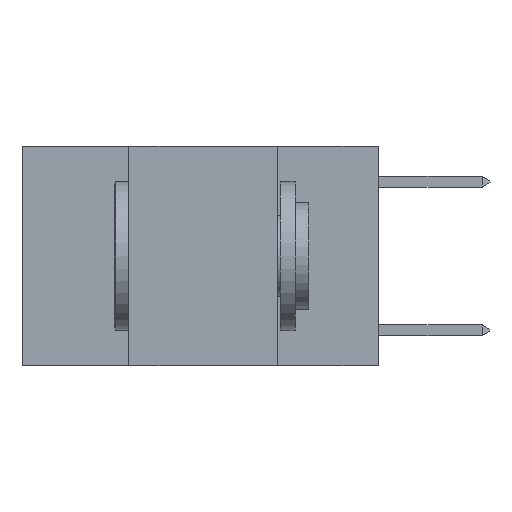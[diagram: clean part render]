
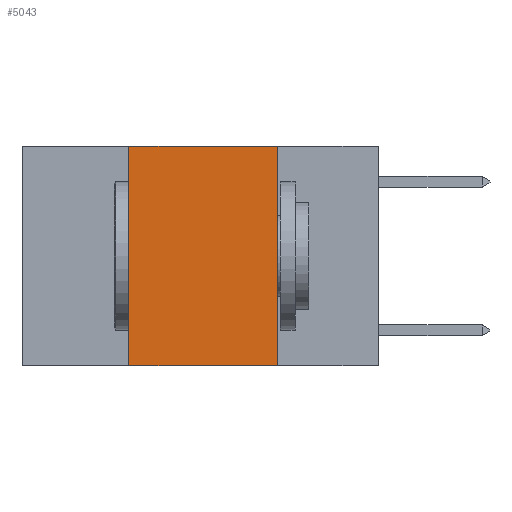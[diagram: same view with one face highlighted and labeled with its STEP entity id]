
A CAD part, left-side view. The second image highlights one B-rep face of the part: STEP entity #5043.
In plain terms, the highlighted planar face has unit normal (-1, 0, 0).
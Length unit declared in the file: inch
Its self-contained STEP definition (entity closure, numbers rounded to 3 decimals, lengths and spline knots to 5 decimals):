
#32 = VECTOR ( 'NONE', #8214, 39.37008 ) ;
#274 = CARTESIAN_POINT ( 'NONE',  ( 0., 0.6, 0. ) ) ;
#342 = VECTOR ( 'NONE', #1905, 39.37008 ) ;
#621 = EDGE_CURVE ( 'NONE', #5665, #5463, #1216, .T. ) ;
#1065 = CARTESIAN_POINT ( 'NONE',  ( 0., 0.42, -0.37 ) ) ;
#1211 = LINE ( 'NONE', #9480, #8311 ) ;
#1216 = LINE ( 'NONE', #7091, #3207 ) ;
#1454 = CARTESIAN_POINT ( 'NONE',  ( 0., 0.17, -0.37 ) ) ;
#1811 = DIRECTION ( 'NONE',  ( 1., 0., 0. ) ) ;
#1905 = DIRECTION ( 'NONE',  ( 0., -1., 0. ) ) ;
#2370 = ORIENTED_EDGE ( 'NONE', *, *, #3875, .F. ) ;
#3207 = VECTOR ( 'NONE', #4194, 39.37008 ) ;
#3368 = CARTESIAN_POINT ( 'NONE',  ( 0., 0.42, 0. ) ) ;
#3630 = ORIENTED_EDGE ( 'NONE', *, *, #9413, .T. ) ;
#3875 = EDGE_CURVE ( 'NONE', #6298, #5665, #1211, .T. ) ;
#4194 = DIRECTION ( 'NONE',  ( 0., -1., 0. ) ) ;
#4341 = ORIENTED_EDGE ( 'NONE', *, *, #9216, .F. ) ;
#4863 = DIRECTION ( 'NONE',  ( 0., 0., 1. ) ) ;
#5043 = ADVANCED_FACE ( 'NONE', ( #6138 ), #6907, .F. ) ;
#5310 = VERTEX_POINT ( 'NONE', #1454 ) ;
#5463 = VERTEX_POINT ( 'NONE', #8295 ) ;
#5513 = ORIENTED_EDGE ( 'NONE', *, *, #621, .F. ) ;
#5665 = VERTEX_POINT ( 'NONE', #3368 ) ;
#5788 = AXIS2_PLACEMENT_3D ( 'NONE', #274, #1811, #9199 ) ;
#6138 = FACE_OUTER_BOUND ( 'NONE', #7334, .T. ) ;
#6288 = LINE ( 'NONE', #8521, #342 ) ;
#6298 = VERTEX_POINT ( 'NONE', #1065 ) ;
#6907 = PLANE ( 'NONE',  #5788 ) ;
#7091 = CARTESIAN_POINT ( 'NONE',  ( 0., 0.6, 0. ) ) ;
#7334 = EDGE_LOOP ( 'NONE', ( #4341, #5513, #2370, #3630 ) ) ;
#7538 = CARTESIAN_POINT ( 'NONE',  ( 0., 0.17, 0. ) ) ;
#8172 = LINE ( 'NONE', #7538, #32 ) ;
#8214 = DIRECTION ( 'NONE',  ( 0., 0., -1. ) ) ;
#8295 = CARTESIAN_POINT ( 'NONE',  ( 0., 0.17, 0. ) ) ;
#8311 = VECTOR ( 'NONE', #4863, 39.37008 ) ;
#8521 = CARTESIAN_POINT ( 'NONE',  ( 0., 0.6, -0.37 ) ) ;
#9199 = DIRECTION ( 'NONE',  ( 0., 0., -1. ) ) ;
#9216 = EDGE_CURVE ( 'NONE', #5463, #5310, #8172, .T. ) ;
#9413 = EDGE_CURVE ( 'NONE', #6298, #5310, #6288, .T. ) ;
#9480 = CARTESIAN_POINT ( 'NONE',  ( 0., 0.42, 0. ) ) ;
